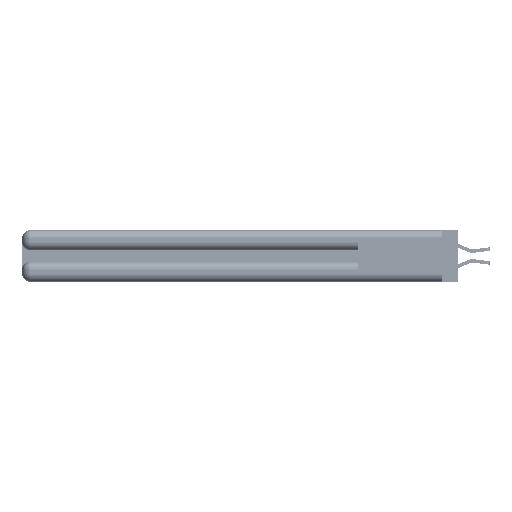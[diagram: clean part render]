
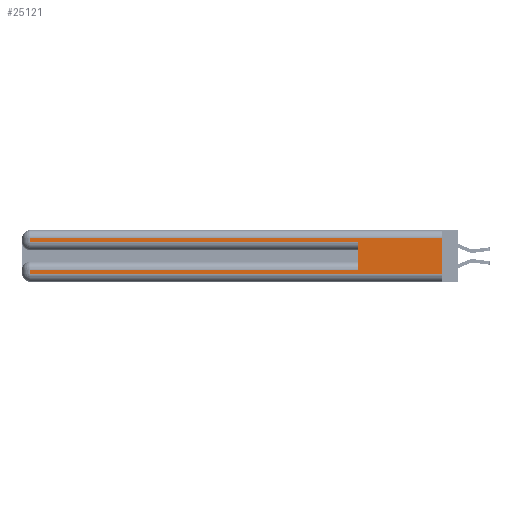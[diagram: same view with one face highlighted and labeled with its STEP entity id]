
A CAD part, left-side view. The second image highlights one B-rep face of the part: STEP entity #25121.
In plain terms, the highlighted planar face has unit normal (-1, 0, 0).
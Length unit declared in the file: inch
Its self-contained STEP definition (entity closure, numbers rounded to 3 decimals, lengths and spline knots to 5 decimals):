
#971 = CARTESIAN_POINT ( 'NONE',  ( 0., 0.6, 0.285 ) ) ;
#1584 = VERTEX_POINT ( 'NONE', #3505 ) ;
#3186 = DIRECTION ( 'NONE',  ( 0., 0., -1. ) ) ;
#3505 = CARTESIAN_POINT ( 'NONE',  ( 0., 0., 0.31 ) ) ;
#3562 = DIRECTION ( 'NONE',  ( 0., 0., -1. ) ) ;
#3899 = DIRECTION ( 'NONE',  ( 1., 0., 0. ) ) ;
#4612 = DIRECTION ( 'NONE',  ( 0., -1., 0. ) ) ;
#5023 = EDGE_CURVE ( 'NONE', #1584, #28895, #24034, .T. ) ;
#5611 = VECTOR ( 'NONE', #3186, 39.37008 ) ;
#6909 = LINE ( 'NONE', #18904, #14871 ) ;
#8301 = CARTESIAN_POINT ( 'NONE',  ( 0., 2.94, 0.37 ) ) ;
#8995 = CARTESIAN_POINT ( 'NONE',  ( 0., 0., 0.06 ) ) ;
#9419 = EDGE_CURVE ( 'NONE', #28895, #20550, #34911, .T. ) ;
#9887 = LINE ( 'NONE', #39479, #32395 ) ;
#11037 = PLANE ( 'NONE',  #24591 ) ;
#12532 = VERTEX_POINT ( 'NONE', #33638 ) ;
#13813 = EDGE_CURVE ( 'NONE', #40767, #49335, #29693, .T. ) ;
#13899 = LINE ( 'NONE', #27940, #29670 ) ;
#14098 = ORIENTED_EDGE ( 'NONE', *, *, #41785, .F. ) ;
#14871 = VECTOR ( 'NONE', #26888, 39.37008 ) ;
#16194 = DIRECTION ( 'NONE',  ( 0., 0., -1. ) ) ;
#16222 = EDGE_CURVE ( 'NONE', #12532, #21185, #13899, .T. ) ;
#16473 = ORIENTED_EDGE ( 'NONE', *, *, #16222, .T. ) ;
#18566 = VECTOR ( 'NONE', #27142, 39.37008 ) ;
#18904 = CARTESIAN_POINT ( 'NONE',  ( 0., 2.94, 0.37 ) ) ;
#19593 = EDGE_CURVE ( 'NONE', #20550, #49335, #9887, .T. ) ;
#19674 = CARTESIAN_POINT ( 'NONE',  ( 0., 0., 0.31 ) ) ;
#20550 = VERTEX_POINT ( 'NONE', #36946 ) ;
#21185 = VERTEX_POINT ( 'NONE', #8995 ) ;
#22796 = CARTESIAN_POINT ( 'NONE',  ( 0., 2.94, 0.085 ) ) ;
#24034 = LINE ( 'NONE', #19674, #18566 ) ;
#24591 = AXIS2_PLACEMENT_3D ( 'NONE', #50304, #3899, #3562 ) ;
#25121 = ADVANCED_FACE ( 'NONE', ( #31057 ), #11037, .F. ) ;
#26277 = DIRECTION ( 'NONE',  ( 0., 0., 1. ) ) ;
#26888 = DIRECTION ( 'NONE',  ( 0., 0., -1. ) ) ;
#27142 = DIRECTION ( 'NONE',  ( 0., 1., 0. ) ) ;
#27251 = EDGE_CURVE ( 'NONE', #40767, #31990, #40079, .T. ) ;
#27940 = CARTESIAN_POINT ( 'NONE',  ( 0., 0., 0.06 ) ) ;
#28343 = CARTESIAN_POINT ( 'NONE',  ( 0., 2.94, 0.31 ) ) ;
#28895 = VERTEX_POINT ( 'NONE', #28343 ) ;
#29669 = DIRECTION ( 'NONE',  ( 0., 1., 0. ) ) ;
#29670 = VECTOR ( 'NONE', #4612, 39.37008 ) ;
#29693 = LINE ( 'NONE', #49668, #32111 ) ;
#30451 = ORIENTED_EDGE ( 'NONE', *, *, #40748, .T. ) ;
#31057 = FACE_OUTER_BOUND ( 'NONE', #36517, .T. ) ;
#31990 = VERTEX_POINT ( 'NONE', #22796 ) ;
#32111 = VECTOR ( 'NONE', #26277, 39.37008 ) ;
#32188 = ORIENTED_EDGE ( 'NONE', *, *, #9419, .T. ) ;
#32395 = VECTOR ( 'NONE', #38990, 39.37008 ) ;
#33638 = CARTESIAN_POINT ( 'NONE',  ( 0., 2.94, 0.06 ) ) ;
#34911 = LINE ( 'NONE', #8301, #48903 ) ;
#35652 = CARTESIAN_POINT ( 'NONE',  ( 0., 0.6, 0.085 ) ) ;
#36438 = VECTOR ( 'NONE', #29669, 39.37008 ) ;
#36517 = EDGE_LOOP ( 'NONE', ( #14098, #40450, #32188, #38925, #45156, #36521, #30451, #16473 ) ) ;
#36521 = ORIENTED_EDGE ( 'NONE', *, *, #27251, .T. ) ;
#36946 = CARTESIAN_POINT ( 'NONE',  ( 0., 2.94, 0.285 ) ) ;
#38453 = LINE ( 'NONE', #45879, #5611 ) ;
#38925 = ORIENTED_EDGE ( 'NONE', *, *, #19593, .T. ) ;
#38990 = DIRECTION ( 'NONE',  ( 0., -1., 0. ) ) ;
#39479 = CARTESIAN_POINT ( 'NONE',  ( 0., 0., 0.285 ) ) ;
#40079 = LINE ( 'NONE', #41172, #36438 ) ;
#40450 = ORIENTED_EDGE ( 'NONE', *, *, #5023, .T. ) ;
#40748 = EDGE_CURVE ( 'NONE', #31990, #12532, #6909, .T. ) ;
#40767 = VERTEX_POINT ( 'NONE', #35652 ) ;
#41172 = CARTESIAN_POINT ( 'NONE',  ( 0., 0., 0.085 ) ) ;
#41785 = EDGE_CURVE ( 'NONE', #1584, #21185, #38453, .T. ) ;
#45156 = ORIENTED_EDGE ( 'NONE', *, *, #13813, .F. ) ;
#45879 = CARTESIAN_POINT ( 'NONE',  ( 0., 0., 0.37 ) ) ;
#48903 = VECTOR ( 'NONE', #16194, 39.37008 ) ;
#49335 = VERTEX_POINT ( 'NONE', #971 ) ;
#49668 = CARTESIAN_POINT ( 'NONE',  ( 0., 0.6, 0.145 ) ) ;
#50304 = CARTESIAN_POINT ( 'NONE',  ( 0., 0., 0.37 ) ) ;
